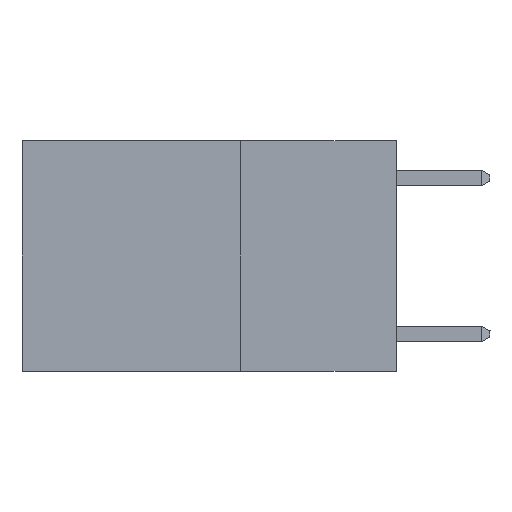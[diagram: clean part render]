
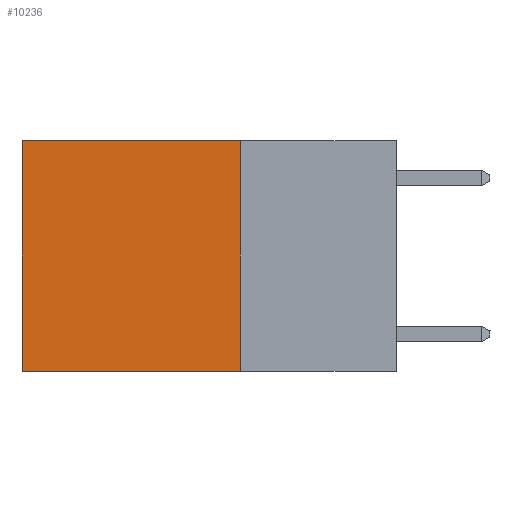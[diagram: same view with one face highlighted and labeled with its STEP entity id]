
A CAD part, left-side view. The second image highlights one B-rep face of the part: STEP entity #10236.
In plain terms, the highlighted planar face has unit normal (-1, 0, 0).
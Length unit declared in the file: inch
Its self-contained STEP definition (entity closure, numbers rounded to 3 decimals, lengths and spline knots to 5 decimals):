
#134 = CARTESIAN_POINT ( 'NONE',  ( 0.2625, 0.6, -0.37 ) ) ;
#417 = PLANE ( 'NONE',  #6945 ) ;
#1260 = CARTESIAN_POINT ( 'NONE',  ( 0.2625, 0.25, -0.37 ) ) ;
#1341 = FACE_OUTER_BOUND ( 'NONE', #9220, .T. ) ;
#1396 = DIRECTION ( 'NONE',  ( 1., 0., 0. ) ) ;
#1598 = VECTOR ( 'NONE', #10044, 39.37008 ) ;
#1848 = VERTEX_POINT ( 'NONE', #5235 ) ;
#2432 = EDGE_CURVE ( 'NONE', #7140, #2869, #10274, .T. ) ;
#2529 = CARTESIAN_POINT ( 'NONE',  ( 0.2625, 0.6, 0. ) ) ;
#2547 = DIRECTION ( 'NONE',  ( 0., 0., -1. ) ) ;
#2615 = CARTESIAN_POINT ( 'NONE',  ( 0.2625, 0.6, 0. ) ) ;
#2717 = ORIENTED_EDGE ( 'NONE', *, *, #2432, .T. ) ;
#2869 = VERTEX_POINT ( 'NONE', #134 ) ;
#3795 = CARTESIAN_POINT ( 'NONE',  ( 0.2625, 0.25, 0. ) ) ;
#3806 = ORIENTED_EDGE ( 'NONE', *, *, #3841, .F. ) ;
#3841 = EDGE_CURVE ( 'NONE', #9332, #1848, #4898, .T. ) ;
#3985 = LINE ( 'NONE', #1260, #1598 ) ;
#4888 = CARTESIAN_POINT ( 'NONE',  ( 0.2625, 0.25, 0. ) ) ;
#4898 = LINE ( 'NONE', #4888, #11374 ) ;
#5235 = CARTESIAN_POINT ( 'NONE',  ( 0.2625, 0.25, -0.37 ) ) ;
#6085 = VECTOR ( 'NONE', #9053, 39.37008 ) ;
#6351 = LINE ( 'NONE', #3795, #6085 ) ;
#6376 = EDGE_CURVE ( 'NONE', #1848, #2869, #3985, .T. ) ;
#6460 = ORIENTED_EDGE ( 'NONE', *, *, #6376, .F. ) ;
#6823 = EDGE_CURVE ( 'NONE', #9332, #7140, #6351, .T. ) ;
#6945 = AXIS2_PLACEMENT_3D ( 'NONE', #10120, #1396, #7664 ) ;
#7140 = VERTEX_POINT ( 'NONE', #2529 ) ;
#7664 = DIRECTION ( 'NONE',  ( 0., 0., -1. ) ) ;
#8110 = ORIENTED_EDGE ( 'NONE', *, *, #6823, .T. ) ;
#8354 = VECTOR ( 'NONE', #2547, 39.37008 ) ;
#9053 = DIRECTION ( 'NONE',  ( 0., 1., 0. ) ) ;
#9218 = DIRECTION ( 'NONE',  ( 0., 0., -1. ) ) ;
#9220 = EDGE_LOOP ( 'NONE', ( #2717, #6460, #3806, #8110 ) ) ;
#9332 = VERTEX_POINT ( 'NONE', #9610 ) ;
#9610 = CARTESIAN_POINT ( 'NONE',  ( 0.2625, 0.25, 0. ) ) ;
#10044 = DIRECTION ( 'NONE',  ( 0., 1., 0. ) ) ;
#10120 = CARTESIAN_POINT ( 'NONE',  ( 0.2625, 0.25, 0. ) ) ;
#10236 = ADVANCED_FACE ( 'NONE', ( #1341 ), #417, .F. ) ;
#10274 = LINE ( 'NONE', #2615, #8354 ) ;
#11374 = VECTOR ( 'NONE', #9218, 39.37008 ) ;
